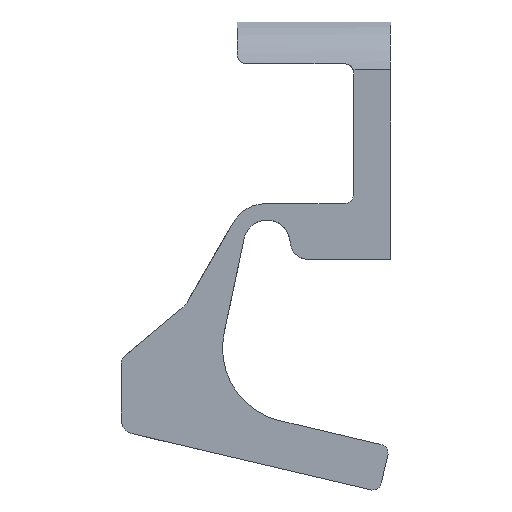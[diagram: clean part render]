
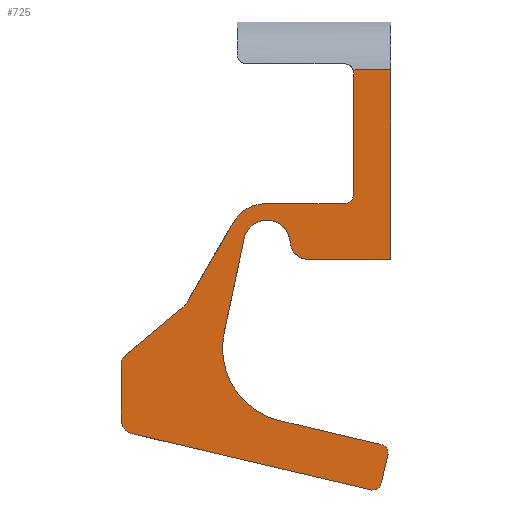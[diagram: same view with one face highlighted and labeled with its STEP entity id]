
A CAD part, left-side view. The second image highlights one B-rep face of the part: STEP entity #725.
In plain terms, the highlighted planar face has unit normal (-1, 0, 0).
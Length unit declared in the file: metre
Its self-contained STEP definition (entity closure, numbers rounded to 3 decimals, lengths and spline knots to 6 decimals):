
#44=CIRCLE('',#772,0.001588);
#45=CIRCLE('',#775,0.001984);
#52=CIRCLE('',#788,0.001191);
#53=CIRCLE('',#791,0.000794);
#54=CIRCLE('',#796,0.003175);
#56=CIRCLE('',#802,0.00635);
#58=CIRCLE('',#806,0.000794);
#60=CIRCLE('',#810,0.000794);
#61=CIRCLE('',#815,0.000794);
#62=CIRCLE('',#816,0.000794);
#63=CIRCLE('',#817,0.001588);
#89=FACE_OUTER_BOUND('',#127,.T.);
#127=EDGE_LOOP('',(#590,#591,#592,#593,#594,#595,#596,#597,#598,#599,#600,
#601,#602,#603,#604,#605,#606,#607,#608,#609,#610,#611,#612));
#152=LINE('',#1056,#220);
#157=LINE('',#1071,#225);
#163=LINE('',#1093,#231);
#166=LINE('',#1101,#234);
#171=LINE('',#1132,#239);
#184=LINE('',#1170,#252);
#188=LINE('',#1182,#256);
#192=LINE('',#1194,#260);
#203=LINE('',#1219,#271);
#207=LINE('',#1231,#275);
#211=LINE('',#1246,#279);
#212=LINE('',#1249,#280);
#220=VECTOR('',#838,0.007888);
#225=VECTOR('',#849,0.010351);
#231=VECTOR('',#867,0.016179);
#234=VECTOR('',#874,0.006995);
#239=VECTOR('',#895,0.008221);
#252=VECTOR('',#930,0.004836);
#256=VECTOR('',#942,0.006494);
#260=VECTOR('',#954,0.006711);
#271=VECTOR('',#977,0.008847);
#275=VECTOR('',#989,0.002381);
#279=VECTOR('',#1005,0.020871);
#280=VECTOR('',#1008,0.003223);
#288=VERTEX_POINT('',#1053);
#289=VERTEX_POINT('',#1055);
#295=VERTEX_POINT('',#1068);
#296=VERTEX_POINT('',#1070);
#305=VERTEX_POINT('',#1090);
#306=VERTEX_POINT('',#1092);
#309=VERTEX_POINT('',#1100);
#311=VERTEX_POINT('',#1115);
#313=VERTEX_POINT('',#1121);
#317=VERTEX_POINT('',#1131);
#329=VERTEX_POINT('',#1163);
#330=VERTEX_POINT('',#1164);
#331=VERTEX_POINT('',#1169);
#332=VERTEX_POINT('',#1173);
#335=VERTEX_POINT('',#1181);
#338=VERTEX_POINT('',#1189);
#339=VERTEX_POINT('',#1193);
#345=VERTEX_POINT('',#1210);
#347=VERTEX_POINT('',#1216);
#349=VERTEX_POINT('',#1222);
#351=VERTEX_POINT('',#1228);
#353=VERTEX_POINT('',#1234);
#357=VERTEX_POINT('',#1248);
#360=EDGE_CURVE('',#288,#289,#152,.T.);
#367=EDGE_CURVE('',#296,#295,#157,.T.);
#377=EDGE_CURVE('',#305,#306,#163,.T.);
#381=EDGE_CURVE('',#306,#309,#166,.T.);
#384=EDGE_CURVE('',#309,#311,#44,.T.);
#387=EDGE_CURVE('',#311,#313,#45,.F.);
#392=EDGE_CURVE('',#313,#317,#171,.T.);
#409=EDGE_CURVE('',#329,#330,#52,.F.);
#412=EDGE_CURVE('',#331,#329,#184,.T.);
#414=EDGE_CURVE('',#332,#331,#53,.F.);
#418=EDGE_CURVE('',#332,#335,#188,.T.);
#422=EDGE_CURVE('',#289,#338,#54,.T.);
#424=EDGE_CURVE('',#339,#338,#192,.T.);
#434=EDGE_CURVE('',#317,#345,#56,.F.);
#437=EDGE_CURVE('',#345,#347,#203,.T.);
#440=EDGE_CURVE('',#347,#349,#58,.T.);
#443=EDGE_CURVE('',#349,#351,#207,.T.);
#446=EDGE_CURVE('',#351,#353,#60,.T.);
#451=EDGE_CURVE('',#353,#330,#211,.T.);
#452=EDGE_CURVE('',#305,#357,#212,.T.);
#453=EDGE_CURVE('',#357,#296,#61,.T.);
#454=EDGE_CURVE('',#295,#339,#62,.T.);
#455=EDGE_CURVE('',#288,#335,#63,.T.);
#590=ORIENTED_EDGE('',*,*,#377,.F.);
#591=ORIENTED_EDGE('',*,*,#452,.T.);
#592=ORIENTED_EDGE('',*,*,#453,.T.);
#593=ORIENTED_EDGE('',*,*,#367,.T.);
#594=ORIENTED_EDGE('',*,*,#454,.T.);
#595=ORIENTED_EDGE('',*,*,#424,.T.);
#596=ORIENTED_EDGE('',*,*,#422,.F.);
#597=ORIENTED_EDGE('',*,*,#360,.F.);
#598=ORIENTED_EDGE('',*,*,#455,.T.);
#599=ORIENTED_EDGE('',*,*,#418,.F.);
#600=ORIENTED_EDGE('',*,*,#414,.T.);
#601=ORIENTED_EDGE('',*,*,#412,.T.);
#602=ORIENTED_EDGE('',*,*,#409,.T.);
#603=ORIENTED_EDGE('',*,*,#451,.F.);
#604=ORIENTED_EDGE('',*,*,#446,.F.);
#605=ORIENTED_EDGE('',*,*,#443,.F.);
#606=ORIENTED_EDGE('',*,*,#440,.F.);
#607=ORIENTED_EDGE('',*,*,#437,.F.);
#608=ORIENTED_EDGE('',*,*,#434,.F.);
#609=ORIENTED_EDGE('',*,*,#392,.F.);
#610=ORIENTED_EDGE('',*,*,#387,.F.);
#611=ORIENTED_EDGE('',*,*,#384,.F.);
#612=ORIENTED_EDGE('',*,*,#381,.F.);
#698=PLANE('',#814);
#725=ADVANCED_FACE('',(#89),#698,.F.);
#772=AXIS2_PLACEMENT_3D('',#1116,#878,#879);
#775=AXIS2_PLACEMENT_3D('',#1122,#885,#886);
#788=AXIS2_PLACEMENT_3D('',#1165,#924,#925);
#791=AXIS2_PLACEMENT_3D('',#1174,#934,#935);
#796=AXIS2_PLACEMENT_3D('',#1190,#949,#950);
#802=AXIS2_PLACEMENT_3D('',#1213,#971,#972);
#806=AXIS2_PLACEMENT_3D('',#1225,#983,#984);
#810=AXIS2_PLACEMENT_3D('',#1237,#995,#996);
#814=AXIS2_PLACEMENT_3D('',#1247,#1006,#1007);
#815=AXIS2_PLACEMENT_3D('',#1250,#1009,#1010);
#816=AXIS2_PLACEMENT_3D('',#1251,#1011,#1012);
#817=AXIS2_PLACEMENT_3D('',#1252,#1013,#1014);
#838=DIRECTION('',(0.,-0.5,0.866));
#849=DIRECTION('',(0.,0.,-1.));
#867=DIRECTION('',(0.,0.,-1.));
#874=DIRECTION('',(0.,1.,0.));
#878=DIRECTION('center_axis',(1.,0.,0.));
#879=DIRECTION('ref_axis',(0.,0.,-1.));
#885=DIRECTION('center_axis',(1.,0.,0.));
#886=DIRECTION('ref_axis',(0.,0.,-1.));
#895=DIRECTION('',(0.,0.208,-0.978));
#924=DIRECTION('center_axis',(1.,0.,0.));
#925=DIRECTION('ref_axis',(0.,0.,-1.));
#930=DIRECTION('',(0.,0.,-1.));
#934=DIRECTION('center_axis',(1.,0.,0.));
#935=DIRECTION('ref_axis',(0.,0.,-1.));
#942=DIRECTION('',(0.,-0.766,0.643));
#949=DIRECTION('center_axis',(1.,0.,0.));
#950=DIRECTION('ref_axis',(0.,0.,-1.));
#954=DIRECTION('',(0.,1.,0.));
#971=DIRECTION('center_axis',(1.,0.,0.));
#972=DIRECTION('ref_axis',(0.,0.,-1.));
#977=DIRECTION('',(0.,-0.973,-0.229));
#983=DIRECTION('center_axis',(1.,0.,0.));
#984=DIRECTION('ref_axis',(0.,0.,-1.));
#989=DIRECTION('',(0.,0.229,-0.973));
#995=DIRECTION('center_axis',(1.,0.,0.));
#996=DIRECTION('ref_axis',(0.,0.,-1.));
#1005=DIRECTION('',(0.,0.973,0.229));
#1006=DIRECTION('center_axis',(1.,0.,0.));
#1007=DIRECTION('ref_axis',(0.,0.,-1.));
#1008=DIRECTION('',(0.,1.,0.));
#1009=DIRECTION('center_axis',(1.,0.,0.));
#1010=DIRECTION('ref_axis',(0.,0.,-1.));
#1011=DIRECTION('center_axis',(1.,0.,0.));
#1012=DIRECTION('ref_axis',(0.,0.,-1.));
#1013=DIRECTION('center_axis',(1.,0.,0.));
#1014=DIRECTION('ref_axis',(0.,0.,-1.));
#1053=CARTESIAN_POINT('',(-0.006223,0.007848,-0.014387));
#1055=CARTESIAN_POINT('',(-0.006223,0.003904,-0.007557));
#1056=CARTESIAN_POINT('',(-0.006223,0.007848,-0.014387));
#1068=CARTESIAN_POINT('',(-0.006223,-0.00635,-0.005175));
#1070=CARTESIAN_POINT('',(-0.006223,-0.00635,0.005175));
#1071=CARTESIAN_POINT('',(-0.006223,-0.00635,0.005175));
#1090=CARTESIAN_POINT('',(-0.006223,-0.009525,0.005447));
#1092=CARTESIAN_POINT('',(-0.006223,-0.009525,-0.010732));
#1093=CARTESIAN_POINT('',(-0.006223,-0.009525,0.005447));
#1100=CARTESIAN_POINT('',(-0.006223,-0.00253,-0.010732));
#1101=CARTESIAN_POINT('',(-0.006223,-0.009525,-0.010732));
#1115=CARTESIAN_POINT('',(-0.006223,-0.000945,-0.009236));
#1116=CARTESIAN_POINT('Origin',(-0.006223,-0.00253,-0.009144));
#1121=CARTESIAN_POINT('',(-0.006223,0.002977,-0.008938));
#1122=CARTESIAN_POINT('Origin',(-0.006223,0.001036,-0.00935));
#1131=CARTESIAN_POINT('',(-0.006223,0.004686,-0.016979));
#1132=CARTESIAN_POINT('',(-0.006223,0.002977,-0.008938));
#1163=CARTESIAN_POINT('',(-0.006223,0.013461,-0.024428));
#1164=CARTESIAN_POINT('',(-0.006223,0.012544,-0.025587));
#1165=CARTESIAN_POINT('Origin',(-0.006223,0.012271,-0.024428));
#1169=CARTESIAN_POINT('',(-0.006223,0.013461,-0.019592));
#1170=CARTESIAN_POINT('',(-0.006223,0.013461,-0.019592));
#1173=CARTESIAN_POINT('',(-0.006223,0.013178,-0.018984));
#1174=CARTESIAN_POINT('Origin',(-0.006223,0.012668,-0.019592));
#1181=CARTESIAN_POINT('',(-0.006223,0.008203,-0.01481));
#1182=CARTESIAN_POINT('',(-0.006223,0.013178,-0.018984));
#1189=CARTESIAN_POINT('',(-0.006223,0.001155,-0.005969));
#1190=CARTESIAN_POINT('Origin',(-0.006223,0.001155,-0.009144));
#1193=CARTESIAN_POINT('',(-0.006223,-0.005556,-0.005969));
#1194=CARTESIAN_POINT('',(-0.006223,-0.005556,-0.005969));
#1210=CARTESIAN_POINT('',(-0.006223,-0.00007,-0.02448));
#1213=CARTESIAN_POINT('Origin',(-0.006223,-0.001525,-0.018299));
#1216=CARTESIAN_POINT('',(-0.006223,-0.008681,-0.026508));
#1219=CARTESIAN_POINT('',(-0.006223,-0.00007,-0.02448));
#1222=CARTESIAN_POINT('',(-0.006223,-0.009272,-0.027462));
#1225=CARTESIAN_POINT('Origin',(-0.006223,-0.008499,-0.02728));
#1228=CARTESIAN_POINT('',(-0.006223,-0.008726,-0.02978));
#1231=CARTESIAN_POINT('',(-0.006223,-0.009272,-0.027462));
#1234=CARTESIAN_POINT('',(-0.006223,-0.007771,-0.030371));
#1237=CARTESIAN_POINT('Origin',(-0.006223,-0.007953,-0.029598));
#1246=CARTESIAN_POINT('',(-0.006223,-0.007771,-0.030371));
#1247=CARTESIAN_POINT('Origin',(-0.006223,0.,0.));
#1248=CARTESIAN_POINT('',(-0.006223,-0.006302,0.005447));
#1249=CARTESIAN_POINT('',(-0.006223,-0.009525,0.005447));
#1250=CARTESIAN_POINT('Origin',(-0.006223,-0.005556,0.005175));
#1251=CARTESIAN_POINT('Origin',(-0.006223,-0.005556,-0.005175));
#1252=CARTESIAN_POINT('Origin',(-0.006223,0.009223,-0.013594));
